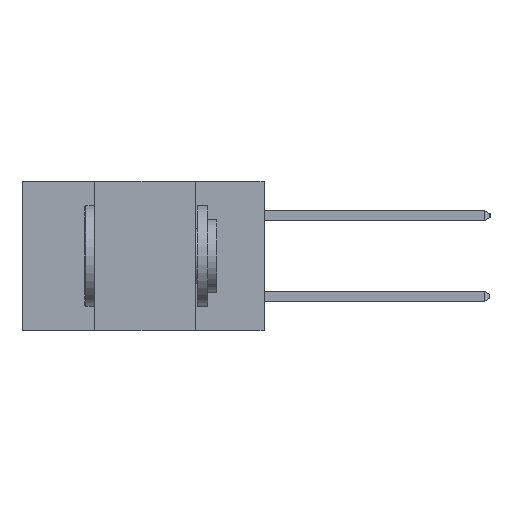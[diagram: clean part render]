
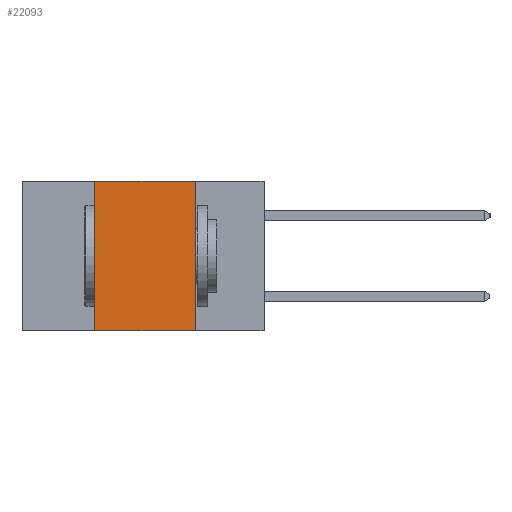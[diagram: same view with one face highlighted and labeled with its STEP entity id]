
A CAD part, left-side view. The second image highlights one B-rep face of the part: STEP entity #22093.
In plain terms, the highlighted planar face has unit normal (-1, 0, 0).
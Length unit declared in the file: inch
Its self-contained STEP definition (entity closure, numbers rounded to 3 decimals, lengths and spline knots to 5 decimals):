
#84 = LINE ( 'NONE', #10819, #4486 ) ;
#206 = DIRECTION ( 'NONE',  ( 0., -1., 0. ) ) ;
#992 = DIRECTION ( 'NONE',  ( 0., 0., -1. ) ) ;
#3799 = EDGE_CURVE ( 'NONE', #13321, #18345, #9979, .T. ) ;
#4486 = VECTOR ( 'NONE', #206, 39.37008 ) ;
#4755 = AXIS2_PLACEMENT_3D ( 'NONE', #21458, #5345, #992 ) ;
#5159 = CARTESIAN_POINT ( 'NONE',  ( 0., 0.42, -0.37 ) ) ;
#5219 = ORIENTED_EDGE ( 'NONE', *, *, #3799, .F. ) ;
#5345 = DIRECTION ( 'NONE',  ( 1., 0., 0. ) ) ;
#5349 = ORIENTED_EDGE ( 'NONE', *, *, #13453, .F. ) ;
#5397 = ORIENTED_EDGE ( 'NONE', *, *, #16578, .T. ) ;
#7107 = PLANE ( 'NONE',  #4755 ) ;
#8220 = CARTESIAN_POINT ( 'NONE',  ( 0., 0.6, 0. ) ) ;
#8238 = CARTESIAN_POINT ( 'NONE',  ( 0., 0.42, -0.37 ) ) ;
#9130 = CARTESIAN_POINT ( 'NONE',  ( 0., 0.17, -0.37 ) ) ;
#9924 = VECTOR ( 'NONE', #18769, 39.37008 ) ;
#9979 = LINE ( 'NONE', #8220, #9924 ) ;
#10819 = CARTESIAN_POINT ( 'NONE',  ( 0., 0.6, -0.37 ) ) ;
#11603 = EDGE_LOOP ( 'NONE', ( #5349, #5219, #18427, #5397 ) ) ;
#11689 = VECTOR ( 'NONE', #13525, 39.37008 ) ;
#11870 = CARTESIAN_POINT ( 'NONE',  ( 0., 0.17, -0.37 ) ) ;
#13321 = VERTEX_POINT ( 'NONE', #19894 ) ;
#13453 = EDGE_CURVE ( 'NONE', #18345, #14309, #20355, .T. ) ;
#13525 = DIRECTION ( 'NONE',  ( 0., 0., 1. ) ) ;
#14309 = VERTEX_POINT ( 'NONE', #9130 ) ;
#14855 = VERTEX_POINT ( 'NONE', #5159 ) ;
#16578 = EDGE_CURVE ( 'NONE', #14855, #14309, #84, .T. ) ;
#18345 = VERTEX_POINT ( 'NONE', #19076 ) ;
#18427 = ORIENTED_EDGE ( 'NONE', *, *, #23206, .F. ) ;
#18769 = DIRECTION ( 'NONE',  ( 0., -1., 0. ) ) ;
#19076 = CARTESIAN_POINT ( 'NONE',  ( 0., 0.17, 0. ) ) ;
#19665 = VECTOR ( 'NONE', #22228, 39.37008 ) ;
#19894 = CARTESIAN_POINT ( 'NONE',  ( 0., 0.42, 0. ) ) ;
#20355 = LINE ( 'NONE', #11870, #19665 ) ;
#21458 = CARTESIAN_POINT ( 'NONE',  ( 0., 0.6, 0. ) ) ;
#21924 = FACE_OUTER_BOUND ( 'NONE', #11603, .T. ) ;
#22093 = ADVANCED_FACE ( 'NONE', ( #21924 ), #7107, .F. ) ;
#22228 = DIRECTION ( 'NONE',  ( 0., 0., -1. ) ) ;
#22689 = LINE ( 'NONE', #8238, #11689 ) ;
#23206 = EDGE_CURVE ( 'NONE', #14855, #13321, #22689, .T. ) ;
